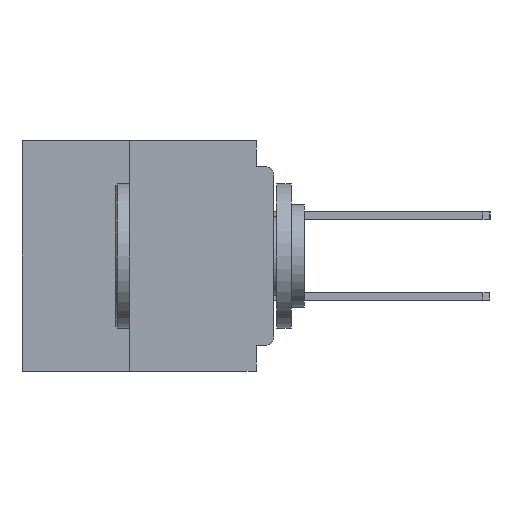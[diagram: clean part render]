
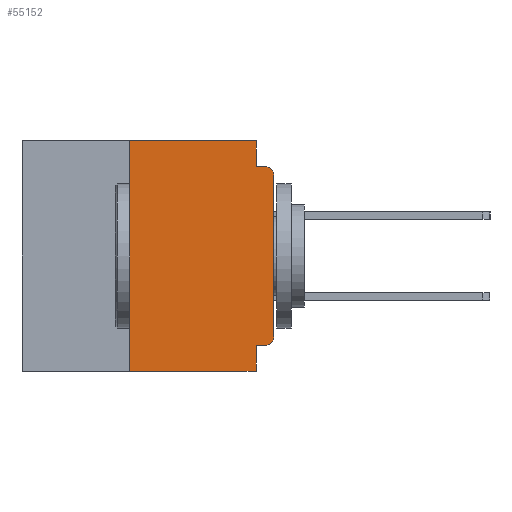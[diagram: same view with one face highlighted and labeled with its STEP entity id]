
A CAD part, left-side view. The second image highlights one B-rep face of the part: STEP entity #55152.
In plain terms, the highlighted planar face has unit normal (-1, 0, 0).
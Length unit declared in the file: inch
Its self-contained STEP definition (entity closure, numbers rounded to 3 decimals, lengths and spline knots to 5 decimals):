
#3385 = EDGE_CURVE ( 'NONE', #19806, #10131, #45736, .T. ) ;
#3993 = VECTOR ( 'NONE', #42950, 39.37008 ) ;
#4293 = ORIENTED_EDGE ( 'NONE', *, *, #37020, .F. ) ;
#5424 = CARTESIAN_POINT ( 'NONE',  ( 0., 0.015, -0.34 ) ) ;
#7342 = VECTOR ( 'NONE', #31335, 39.37008 ) ;
#7388 = ORIENTED_EDGE ( 'NONE', *, *, #44939, .F. ) ;
#7669 = ORIENTED_EDGE ( 'NONE', *, *, #48824, .F. ) ;
#9545 = VERTEX_POINT ( 'NONE', #32414 ) ;
#9690 = CIRCLE ( 'NONE', #28647, 0.015 ) ;
#9881 = EDGE_LOOP ( 'NONE', ( #25399, #41364, #43980, #26908, #7669, #61376, #20491, #7388, #4293, #13168 ) ) ;
#10131 = VERTEX_POINT ( 'NONE', #51780 ) ;
#10334 = DIRECTION ( 'NONE',  ( 0., 0., -1. ) ) ;
#10391 = EDGE_CURVE ( 'NONE', #10131, #34259, #43640, .T. ) ;
#10906 = CARTESIAN_POINT ( 'NONE',  ( 0., 0.015, -0.06 ) ) ;
#12276 = AXIS2_PLACEMENT_3D ( 'NONE', #10906, #44087, #15660 ) ;
#12504 = DIRECTION ( 'NONE',  ( 0., 0., -1. ) ) ;
#13168 = ORIENTED_EDGE ( 'NONE', *, *, #48547, .T. ) ;
#13614 = VECTOR ( 'NONE', #52797, 39.37008 ) ;
#14046 = VERTEX_POINT ( 'NONE', #22721 ) ;
#15660 = DIRECTION ( 'NONE',  ( 0., 0., -1. ) ) ;
#15990 = LINE ( 'NONE', #59751, #39756 ) ;
#16318 = EDGE_CURVE ( 'NONE', #14046, #60655, #18333, .T. ) ;
#17067 = CARTESIAN_POINT ( 'NONE',  ( 0., 0.437, 0. ) ) ;
#18333 = LINE ( 'NONE', #26743, #31020 ) ;
#19354 = CARTESIAN_POINT ( 'NONE',  ( 0., 0.437, -0.4 ) ) ;
#19806 = VERTEX_POINT ( 'NONE', #51004 ) ;
#20491 = ORIENTED_EDGE ( 'NONE', *, *, #41738, .T. ) ;
#22721 = CARTESIAN_POINT ( 'NONE',  ( 0., 0.25, -0.4 ) ) ;
#24772 = VERTEX_POINT ( 'NONE', #39790 ) ;
#24839 = CARTESIAN_POINT ( 'NONE',  ( 0., 0.25, 0. ) ) ;
#25383 = CARTESIAN_POINT ( 'NONE',  ( 0., 0.031, -0.4 ) ) ;
#25399 = ORIENTED_EDGE ( 'NONE', *, *, #3385, .T. ) ;
#26743 = CARTESIAN_POINT ( 'NONE',  ( 0., 0.25, -0.4 ) ) ;
#26908 = ORIENTED_EDGE ( 'NONE', *, *, #52462, .F. ) ;
#27251 = VERTEX_POINT ( 'NONE', #45798 ) ;
#28647 = AXIS2_PLACEMENT_3D ( 'NONE', #5424, #38797, #10334 ) ;
#29311 = CARTESIAN_POINT ( 'NONE',  ( 0., 0.015, -0.045 ) ) ;
#30135 = DIRECTION ( 'NONE',  ( 0., 0., -1. ) ) ;
#30529 = VERTEX_POINT ( 'NONE', #48173 ) ;
#31020 = VECTOR ( 'NONE', #31503, 39.37008 ) ;
#31274 = LINE ( 'NONE', #59536, #7342 ) ;
#31335 = DIRECTION ( 'NONE',  ( 0., -1., 0. ) ) ;
#31503 = DIRECTION ( 'NONE',  ( 0., 0., 1. ) ) ;
#32414 = CARTESIAN_POINT ( 'NONE',  ( 0., 0.031, -0.355 ) ) ;
#33996 = CARTESIAN_POINT ( 'NONE',  ( 0., 0., -0.355 ) ) ;
#34259 = VERTEX_POINT ( 'NONE', #29311 ) ;
#34639 = VECTOR ( 'NONE', #51252, 39.37008 ) ;
#36013 = FACE_OUTER_BOUND ( 'NONE', #9881, .T. ) ;
#36076 = LINE ( 'NONE', #25383, #59662 ) ;
#36177 = PLANE ( 'NONE',  #48136 ) ;
#36279 = DIRECTION ( 'NONE',  ( 0., -1., 0. ) ) ;
#37020 = EDGE_CURVE ( 'NONE', #38199, #9545, #52944, .T. ) ;
#38199 = VERTEX_POINT ( 'NONE', #57668 ) ;
#38797 = DIRECTION ( 'NONE',  ( -1., 0., 0. ) ) ;
#39756 = VECTOR ( 'NONE', #36279, 39.37008 ) ;
#39790 = CARTESIAN_POINT ( 'NONE',  ( 0., 0.031, -0.045 ) ) ;
#40926 = DIRECTION ( 'NONE',  ( 1., 0., 0. ) ) ;
#41364 = ORIENTED_EDGE ( 'NONE', *, *, #10391, .T. ) ;
#41738 = EDGE_CURVE ( 'NONE', #14046, #30529, #54610, .T. ) ;
#42950 = DIRECTION ( 'NONE',  ( 0., -1., 0. ) ) ;
#43640 = CIRCLE ( 'NONE', #12276, 0.015 ) ;
#43786 = VECTOR ( 'NONE', #53991, 39.37008 ) ;
#43980 = ORIENTED_EDGE ( 'NONE', *, *, #45133, .F. ) ;
#44087 = DIRECTION ( 'NONE',  ( -1., 0., 0. ) ) ;
#44487 = CARTESIAN_POINT ( 'NONE',  ( 0., 0.031, 0. ) ) ;
#44939 = EDGE_CURVE ( 'NONE', #9545, #30529, #36076, .T. ) ;
#45133 = EDGE_CURVE ( 'NONE', #24772, #34259, #15990, .T. ) ;
#45736 = LINE ( 'NONE', #51175, #34639 ) ;
#45798 = CARTESIAN_POINT ( 'NONE',  ( 0., 0.031, 0. ) ) ;
#48136 = AXIS2_PLACEMENT_3D ( 'NONE', #17067, #40926, #12504 ) ;
#48173 = CARTESIAN_POINT ( 'NONE',  ( 0., 0.031, -0.4 ) ) ;
#48547 = EDGE_CURVE ( 'NONE', #38199, #19806, #9690, .T. ) ;
#48824 = EDGE_CURVE ( 'NONE', #60655, #27251, #31274, .T. ) ;
#51004 = CARTESIAN_POINT ( 'NONE',  ( 0., 0., -0.34 ) ) ;
#51175 = CARTESIAN_POINT ( 'NONE',  ( 0., 0., 0. ) ) ;
#51252 = DIRECTION ( 'NONE',  ( 0., 0., 1. ) ) ;
#51780 = CARTESIAN_POINT ( 'NONE',  ( 0., 0., -0.06 ) ) ;
#52462 = EDGE_CURVE ( 'NONE', #27251, #24772, #56317, .T. ) ;
#52797 = DIRECTION ( 'NONE',  ( 0., 1., 0. ) ) ;
#52944 = LINE ( 'NONE', #33996, #13614 ) ;
#53991 = DIRECTION ( 'NONE',  ( 0., 0., -1. ) ) ;
#54610 = LINE ( 'NONE', #19354, #3993 ) ;
#55152 = ADVANCED_FACE ( 'NONE', ( #36013 ), #36177, .F. ) ;
#56317 = LINE ( 'NONE', #44487, #43786 ) ;
#57668 = CARTESIAN_POINT ( 'NONE',  ( 0., 0.015, -0.355 ) ) ;
#59536 = CARTESIAN_POINT ( 'NONE',  ( 0., 0.437, 0. ) ) ;
#59662 = VECTOR ( 'NONE', #30135, 39.37008 ) ;
#59751 = CARTESIAN_POINT ( 'NONE',  ( 0., 0., -0.045 ) ) ;
#60655 = VERTEX_POINT ( 'NONE', #24839 ) ;
#61376 = ORIENTED_EDGE ( 'NONE', *, *, #16318, .F. ) ;
